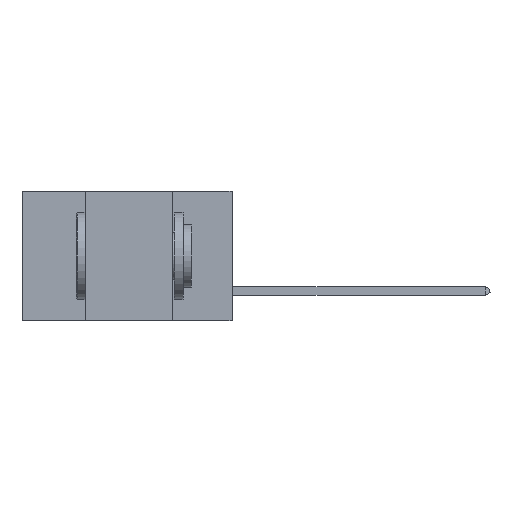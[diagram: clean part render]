
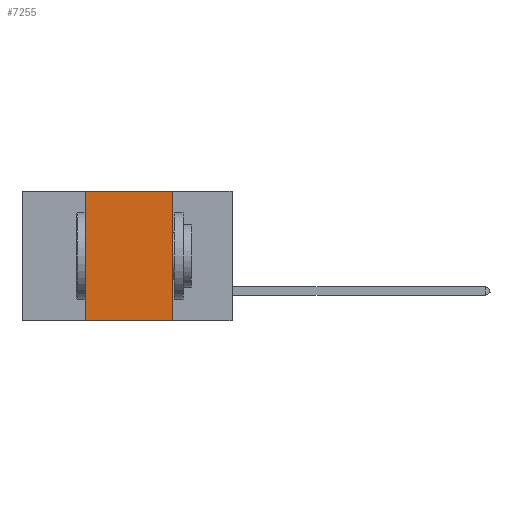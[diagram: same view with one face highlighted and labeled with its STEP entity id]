
A CAD part, left-side view. The second image highlights one B-rep face of the part: STEP entity #7255.
In plain terms, the highlighted planar face has unit normal (-1, 0, 0).
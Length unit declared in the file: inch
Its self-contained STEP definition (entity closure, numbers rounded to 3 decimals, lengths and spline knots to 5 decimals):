
#11 = DIRECTION ( 'NONE',  ( 0., 0., 1. ) ) ;
#657 = ORIENTED_EDGE ( 'NONE', *, *, #5329, .F. ) ;
#733 = LINE ( 'NONE', #24356, #4119 ) ;
#1398 = EDGE_LOOP ( 'NONE', ( #657, #21928, #26954, #15656 ) ) ;
#2877 = VERTEX_POINT ( 'NONE', #38714 ) ;
#4119 = VECTOR ( 'NONE', #9156, 39.37008 ) ;
#5024 = VERTEX_POINT ( 'NONE', #46984 ) ;
#5329 = EDGE_CURVE ( 'NONE', #45850, #5024, #12732, .T. ) ;
#6917 = FACE_OUTER_BOUND ( 'NONE', #1398, .T. ) ;
#7252 = VECTOR ( 'NONE', #17115, 39.37008 ) ;
#7255 = ADVANCED_FACE ( 'NONE', ( #6917 ), #32996, .F. ) ;
#8592 = CARTESIAN_POINT ( 'NONE',  ( 0., 0.6, -0.37 ) ) ;
#8928 = CARTESIAN_POINT ( 'NONE',  ( 0., 0.17, 0. ) ) ;
#9156 = DIRECTION ( 'NONE',  ( 0., -1., 0. ) ) ;
#10614 = CARTESIAN_POINT ( 'NONE',  ( 0., 0.42, 0. ) ) ;
#11562 = VECTOR ( 'NONE', #19494, 39.37008 ) ;
#12732 = LINE ( 'NONE', #23833, #11562 ) ;
#13516 = LINE ( 'NONE', #17969, #15744 ) ;
#14794 = CARTESIAN_POINT ( 'NONE',  ( 0., 0.6, 0. ) ) ;
#15656 = ORIENTED_EDGE ( 'NONE', *, *, #33503, .T. ) ;
#15744 = VECTOR ( 'NONE', #11, 39.37008 ) ;
#17115 = DIRECTION ( 'NONE',  ( 0., -1., 0. ) ) ;
#17969 = CARTESIAN_POINT ( 'NONE',  ( 0., 0.42, 0. ) ) ;
#19494 = DIRECTION ( 'NONE',  ( 0., 0., -1. ) ) ;
#21928 = ORIENTED_EDGE ( 'NONE', *, *, #43283, .F. ) ;
#23833 = CARTESIAN_POINT ( 'NONE',  ( 0., 0.17, 0. ) ) ;
#24356 = CARTESIAN_POINT ( 'NONE',  ( 0., 0.6, 0. ) ) ;
#26954 = ORIENTED_EDGE ( 'NONE', *, *, #45956, .F. ) ;
#29791 = DIRECTION ( 'NONE',  ( 0., 0., -1. ) ) ;
#31905 = VERTEX_POINT ( 'NONE', #10614 ) ;
#32996 = PLANE ( 'NONE',  #33120 ) ;
#33120 = AXIS2_PLACEMENT_3D ( 'NONE', #14794, #41060, #29791 ) ;
#33503 = EDGE_CURVE ( 'NONE', #2877, #5024, #42658, .T. ) ;
#38714 = CARTESIAN_POINT ( 'NONE',  ( 0., 0.42, -0.37 ) ) ;
#41060 = DIRECTION ( 'NONE',  ( 1., 0., 0. ) ) ;
#42658 = LINE ( 'NONE', #8592, #7252 ) ;
#43283 = EDGE_CURVE ( 'NONE', #31905, #45850, #733, .T. ) ;
#45850 = VERTEX_POINT ( 'NONE', #8928 ) ;
#45956 = EDGE_CURVE ( 'NONE', #2877, #31905, #13516, .T. ) ;
#46984 = CARTESIAN_POINT ( 'NONE',  ( 0., 0.17, -0.37 ) ) ;
